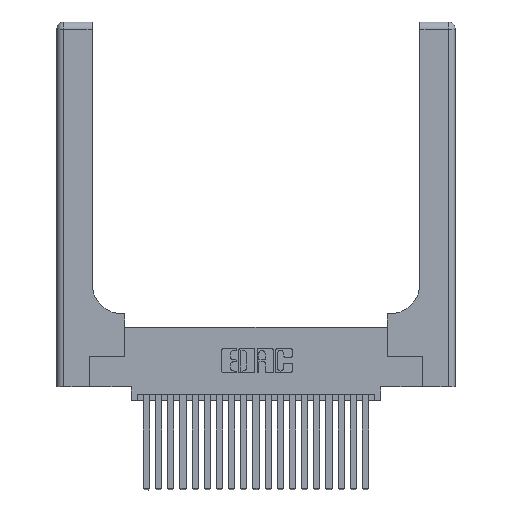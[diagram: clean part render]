
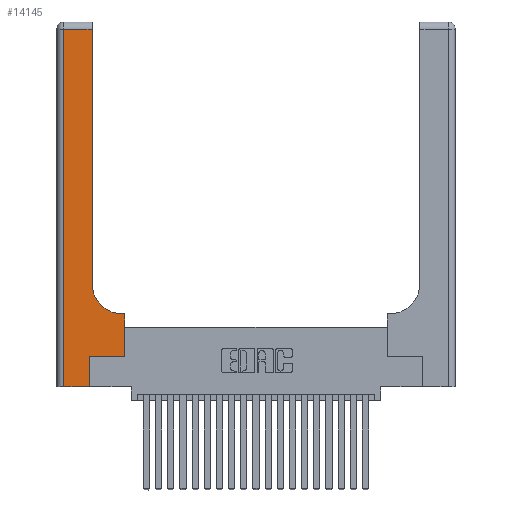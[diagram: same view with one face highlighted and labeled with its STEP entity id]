
A CAD part, top view. The second image highlights one B-rep face of the part: STEP entity #14145.
In plain terms, the highlighted planar face has unit normal (0, 0, 1).
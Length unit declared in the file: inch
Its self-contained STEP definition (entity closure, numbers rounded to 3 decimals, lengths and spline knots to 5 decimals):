
#112 = DIRECTION ( 'NONE',  ( 0., 1., 0. ) ) ;
#314 = EDGE_CURVE ( 'NONE', #20225, #1108, #17549, .T. ) ;
#942 = DIRECTION ( 'NONE',  ( 1., 0., 0. ) ) ;
#1108 = VERTEX_POINT ( 'NONE', #4586 ) ;
#1192 = VECTOR ( 'NONE', #942, 39.37008 ) ;
#2833 = CARTESIAN_POINT ( 'NONE',  ( 0., 3., 0.37 ) ) ;
#2963 = VERTEX_POINT ( 'NONE', #11651 ) ;
#3177 = VECTOR ( 'NONE', #15830, 39.37008 ) ;
#3719 = LINE ( 'NONE', #16596, #14650 ) ;
#4476 = ORIENTED_EDGE ( 'NONE', *, *, #20370, .T. ) ;
#4586 = CARTESIAN_POINT ( 'NONE',  ( 0.06, 2.94, 0.37 ) ) ;
#4875 = DIRECTION ( 'NONE',  ( 1., 0., 0. ) ) ;
#5122 = DIRECTION ( 'NONE',  ( 1., 0., 0. ) ) ;
#5467 = ORIENTED_EDGE ( 'NONE', *, *, #10897, .T. ) ;
#7395 = CARTESIAN_POINT ( 'NONE',  ( 0.06, 3., 0.37 ) ) ;
#8177 = LINE ( 'NONE', #10797, #8749 ) ;
#8368 = EDGE_CURVE ( 'NONE', #14163, #8450, #11524, .T. ) ;
#8450 = VERTEX_POINT ( 'NONE', #19450 ) ;
#8749 = VECTOR ( 'NONE', #112, 39.37008 ) ;
#9063 = LINE ( 'NONE', #11850, #3177 ) ;
#9194 = ORIENTED_EDGE ( 'NONE', *, *, #22030, .T. ) ;
#9201 = CARTESIAN_POINT ( 'NONE',  ( 0.2915, 0.85, 0.37 ) ) ;
#9247 = VECTOR ( 'NONE', #16249, 39.37008 ) ;
#9368 = ORIENTED_EDGE ( 'NONE', *, *, #13304, .T. ) ;
#9886 = AXIS2_PLACEMENT_3D ( 'NONE', #2833, #13655, #22693 ) ;
#10012 = ORIENTED_EDGE ( 'NONE', *, *, #15358, .T. ) ;
#10018 = DIRECTION ( 'NONE',  ( 0., 0., -1. ) ) ;
#10201 = DIRECTION ( 'NONE',  ( -1., 0., 0. ) ) ;
#10456 = LINE ( 'NONE', #23016, #12167 ) ;
#10797 = CARTESIAN_POINT ( 'NONE',  ( 0.269, 0., 0.37 ) ) ;
#10897 = EDGE_CURVE ( 'NONE', #22039, #20225, #9063, .T. ) ;
#11029 = ORIENTED_EDGE ( 'NONE', *, *, #20478, .T. ) ;
#11524 = LINE ( 'NONE', #15173, #1192 ) ;
#11651 = CARTESIAN_POINT ( 'NONE',  ( 0.269, 0., 0.37 ) ) ;
#11850 = CARTESIAN_POINT ( 'NONE',  ( 0.2915, 3., 0.37 ) ) ;
#11855 = ORIENTED_EDGE ( 'NONE', *, *, #314, .T. ) ;
#12167 = VECTOR ( 'NONE', #5122, 39.37008 ) ;
#12524 = CARTESIAN_POINT ( 'NONE',  ( 0., 2.94, 0.37 ) ) ;
#13304 = EDGE_CURVE ( 'NONE', #16784, #22039, #14872, .T. ) ;
#13655 = DIRECTION ( 'NONE',  ( 0., 0., -1. ) ) ;
#13735 = CARTESIAN_POINT ( 'NONE',  ( 0.269, 0.25, 0.37 ) ) ;
#14104 = CARTESIAN_POINT ( 'NONE',  ( 0.2915, 2.94, 0.37 ) ) ;
#14145 = ADVANCED_FACE ( 'NONE', ( #22371 ), #18942, .F. ) ;
#14163 = VERTEX_POINT ( 'NONE', #13735 ) ;
#14237 = DIRECTION ( 'NONE',  ( -1., 0., 0. ) ) ;
#14650 = VECTOR ( 'NONE', #16517, 39.37008 ) ;
#14872 = CIRCLE ( 'NONE', #18867, 0.25 ) ;
#14876 = CARTESIAN_POINT ( 'NONE',  ( 0.5415, 0.6, 0.37 ) ) ;
#15173 = CARTESIAN_POINT ( 'NONE',  ( 0.269, 0.25, 0.37 ) ) ;
#15358 = EDGE_CURVE ( 'NONE', #18767, #16784, #20333, .T. ) ;
#15474 = CARTESIAN_POINT ( 'NONE',  ( 0.2915, 0.6, 0.37 ) ) ;
#15830 = DIRECTION ( 'NONE',  ( 0., 1., 0. ) ) ;
#15964 = ORIENTED_EDGE ( 'NONE', *, *, #8368, .T. ) ;
#16249 = DIRECTION ( 'NONE',  ( 0., -1., 0. ) ) ;
#16517 = DIRECTION ( 'NONE',  ( 0., 1., 0. ) ) ;
#16596 = CARTESIAN_POINT ( 'NONE',  ( 0.5585, 0.25, 0.37 ) ) ;
#16784 = VERTEX_POINT ( 'NONE', #14876 ) ;
#17319 = CARTESIAN_POINT ( 'NONE',  ( 0.5415, 0.85, 0.37 ) ) ;
#17364 = CARTESIAN_POINT ( 'NONE',  ( 0.5585, 0.6, 0.37 ) ) ;
#17549 = LINE ( 'NONE', #12524, #19501 ) ;
#18097 = ORIENTED_EDGE ( 'NONE', *, *, #19456, .T. ) ;
#18767 = VERTEX_POINT ( 'NONE', #17364 ) ;
#18867 = AXIS2_PLACEMENT_3D ( 'NONE', #17319, #10018, #4875 ) ;
#18942 = PLANE ( 'NONE',  #9886 ) ;
#19450 = CARTESIAN_POINT ( 'NONE',  ( 0.5585, 0.25, 0.37 ) ) ;
#19456 = EDGE_CURVE ( 'NONE', #20330, #2963, #10456, .T. ) ;
#19501 = VECTOR ( 'NONE', #14237, 39.37008 ) ;
#19874 = CARTESIAN_POINT ( 'NONE',  ( 0.06, 0., 0.37 ) ) ;
#20225 = VERTEX_POINT ( 'NONE', #14104 ) ;
#20330 = VERTEX_POINT ( 'NONE', #19874 ) ;
#20333 = LINE ( 'NONE', #15474, #22018 ) ;
#20370 = EDGE_CURVE ( 'NONE', #2963, #14163, #8177, .T. ) ;
#20478 = EDGE_CURVE ( 'NONE', #8450, #18767, #3719, .T. ) ;
#21563 = LINE ( 'NONE', #7395, #9247 ) ;
#21632 = EDGE_LOOP ( 'NONE', ( #5467, #11855, #9194, #18097, #4476, #15964, #11029, #10012, #9368 ) ) ;
#22018 = VECTOR ( 'NONE', #10201, 39.37008 ) ;
#22030 = EDGE_CURVE ( 'NONE', #1108, #20330, #21563, .T. ) ;
#22039 = VERTEX_POINT ( 'NONE', #9201 ) ;
#22371 = FACE_OUTER_BOUND ( 'NONE', #21632, .T. ) ;
#22693 = DIRECTION ( 'NONE',  ( -1., 0., 0. ) ) ;
#23016 = CARTESIAN_POINT ( 'NONE',  ( 0., 0., 0.37 ) ) ;
